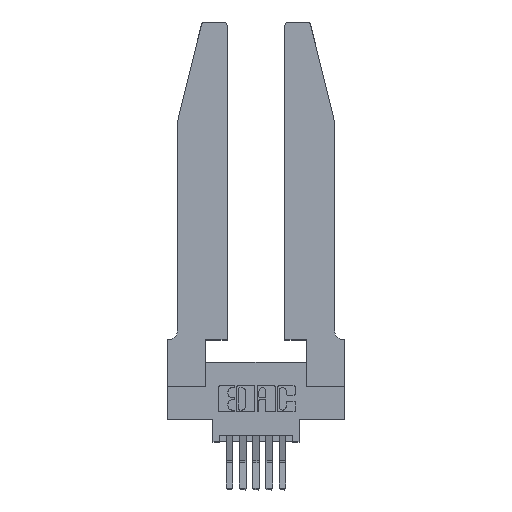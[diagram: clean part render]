
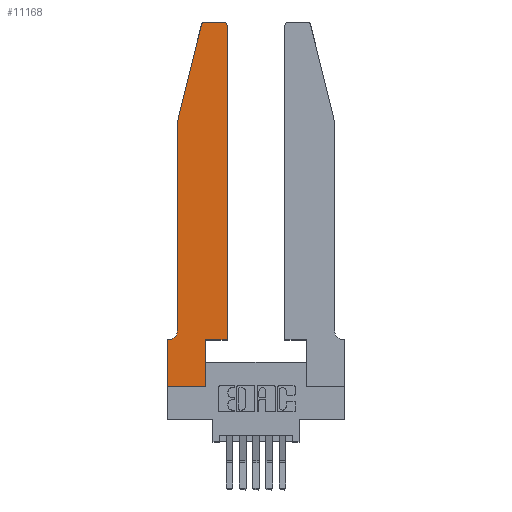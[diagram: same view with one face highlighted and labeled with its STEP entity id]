
A CAD part, top view. The second image highlights one B-rep face of the part: STEP entity #11168.
In plain terms, the highlighted planar face has unit normal (0, 0, 1).
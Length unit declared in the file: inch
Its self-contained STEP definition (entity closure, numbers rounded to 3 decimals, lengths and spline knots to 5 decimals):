
#159 = AXIS2_PLACEMENT_3D ( 'NONE', #1647, #2772, #8067 ) ;
#267 = VECTOR ( 'NONE', #5500, 39.37008 ) ;
#346 = CARTESIAN_POINT ( 'NONE',  ( 0., 0.35, 0.37 ) ) ;
#386 = CARTESIAN_POINT ( 'NONE',  ( 0., 0., 0.37 ) ) ;
#785 = CARTESIAN_POINT ( 'NONE',  ( 0.4205, 2.75, 0.37 ) ) ;
#828 = PLANE ( 'NONE',  #159 ) ;
#939 = ORIENTED_EDGE ( 'NONE', *, *, #6567, .T. ) ;
#1120 = ORIENTED_EDGE ( 'NONE', *, *, #12400, .T. ) ;
#1307 = EDGE_CURVE ( 'NONE', #7925, #9854, #4342, .T. ) ;
#1395 = CARTESIAN_POINT ( 'NONE',  ( 0.4505, 0.35, 0.37 ) ) ;
#1407 = DIRECTION ( 'NONE',  ( 0., 1., 0. ) ) ;
#1647 = CARTESIAN_POINT ( 'NONE',  ( 0., 0.35, 0.37 ) ) ;
#1741 = VERTEX_POINT ( 'NONE', #12977 ) ;
#1859 = AXIS2_PLACEMENT_3D ( 'NONE', #12601, #13687, #10317 ) ;
#1893 = CIRCLE ( 'NONE', #5545, 0.07 ) ;
#1954 = CARTESIAN_POINT ( 'NONE',  ( 0.0755, 0.42, 0.37 ) ) ;
#2406 = ORIENTED_EDGE ( 'NONE', *, *, #13026, .T. ) ;
#2427 = FACE_OUTER_BOUND ( 'NONE', #3702, .T. ) ;
#2658 = VECTOR ( 'NONE', #3907, 39.37008 ) ;
#2772 = DIRECTION ( 'NONE',  ( 0., 0., 1. ) ) ;
#2905 = CARTESIAN_POINT ( 'NONE',  ( 0.0755, 2., 0.37 ) ) ;
#2915 = VECTOR ( 'NONE', #4854, 39.37008 ) ;
#2920 = AXIS2_PLACEMENT_3D ( 'NONE', #3860, #5996, #12474 ) ;
#2990 = ORIENTED_EDGE ( 'NONE', *, *, #1307, .T. ) ;
#3074 = ORIENTED_EDGE ( 'NONE', *, *, #8545, .T. ) ;
#3184 = CARTESIAN_POINT ( 'NONE',  ( 0.4505, 0.35, 0.37 ) ) ;
#3205 = ORIENTED_EDGE ( 'NONE', *, *, #9961, .T. ) ;
#3292 = LINE ( 'NONE', #6955, #13682 ) ;
#3400 = ORIENTED_EDGE ( 'NONE', *, *, #11657, .T. ) ;
#3604 = CARTESIAN_POINT ( 'NONE',  ( 0.2865, 0.35, 0.37 ) ) ;
#3702 = EDGE_LOOP ( 'NONE', ( #10609, #3205, #7312, #8135, #3074, #1120, #2990, #3823, #939, #12648, #2406, #3400 ) ) ;
#3823 = ORIENTED_EDGE ( 'NONE', *, *, #11469, .T. ) ;
#3860 = CARTESIAN_POINT ( 'NONE',  ( 0.284, 2.72, 0.37 ) ) ;
#3907 = DIRECTION ( 'NONE',  ( 0., -1., 0. ) ) ;
#4028 = DIRECTION ( 'NONE',  ( 0., 1., 0. ) ) ;
#4201 = CARTESIAN_POINT ( 'NONE',  ( 0.0055, 0.42, 0.37 ) ) ;
#4342 = LINE ( 'NONE', #8111, #2658 ) ;
#4854 = DIRECTION ( 'NONE',  ( -1., 0., 0. ) ) ;
#5061 = LINE ( 'NONE', #13356, #8101 ) ;
#5265 = CARTESIAN_POINT ( 'NONE',  ( 0.2865, 0.35, 0.37 ) ) ;
#5500 = DIRECTION ( 'NONE',  ( 1., 0., 0. ) ) ;
#5545 = AXIS2_PLACEMENT_3D ( 'NONE', #4201, #5985, #7476 ) ;
#5696 = CARTESIAN_POINT ( 'NONE',  ( 0.0755, 0.35, 0.37 ) ) ;
#5869 = CARTESIAN_POINT ( 'NONE',  ( 0.2605, 2.75, 0.37 ) ) ;
#5920 = VERTEX_POINT ( 'NONE', #1395 ) ;
#5985 = DIRECTION ( 'NONE',  ( 0., 0., -1. ) ) ;
#5996 = DIRECTION ( 'NONE',  ( 0., 0., 1. ) ) ;
#6066 = LINE ( 'NONE', #5696, #12959 ) ;
#6400 = VERTEX_POINT ( 'NONE', #13180 ) ;
#6419 = DIRECTION ( 'NONE',  ( 1., 0., 0. ) ) ;
#6444 = VERTEX_POINT ( 'NONE', #13510 ) ;
#6567 = EDGE_CURVE ( 'NONE', #6400, #8113, #13697, .T. ) ;
#6667 = VERTEX_POINT ( 'NONE', #13475 ) ;
#6842 = EDGE_CURVE ( 'NONE', #11203, #7207, #3292, .T. ) ;
#6850 = CARTESIAN_POINT ( 'NONE',  ( 0.284, 2.75, 0.37 ) ) ;
#6955 = CARTESIAN_POINT ( 'NONE',  ( 0.0755, 2., 0.37 ) ) ;
#7089 = EDGE_CURVE ( 'NONE', #8657, #8095, #8960, .T. ) ;
#7207 = VERTEX_POINT ( 'NONE', #1954 ) ;
#7312 = ORIENTED_EDGE ( 'NONE', *, *, #12575, .T. ) ;
#7476 = DIRECTION ( 'NONE',  ( -1., 0., 0. ) ) ;
#7925 = VERTEX_POINT ( 'NONE', #346 ) ;
#8067 = DIRECTION ( 'NONE',  ( 1., 0., 0. ) ) ;
#8095 = VERTEX_POINT ( 'NONE', #6850 ) ;
#8101 = VECTOR ( 'NONE', #1407, 39.37008 ) ;
#8111 = CARTESIAN_POINT ( 'NONE',  ( 0., 0., 0.37 ) ) ;
#8113 = VERTEX_POINT ( 'NONE', #3604 ) ;
#8119 = LINE ( 'NONE', #8670, #8792 ) ;
#8135 = ORIENTED_EDGE ( 'NONE', *, *, #6842, .T. ) ;
#8545 = EDGE_CURVE ( 'NONE', #7207, #6444, #1893, .T. ) ;
#8657 = VERTEX_POINT ( 'NONE', #785 ) ;
#8670 = CARTESIAN_POINT ( 'NONE',  ( 0., 0., 0.37 ) ) ;
#8792 = VECTOR ( 'NONE', #6419, 39.37008 ) ;
#8960 = LINE ( 'NONE', #5869, #2915 ) ;
#9854 = VERTEX_POINT ( 'NONE', #386 ) ;
#9961 = EDGE_CURVE ( 'NONE', #8095, #6667, #11938, .T. ) ;
#10291 = VECTOR ( 'NONE', #12720, 39.37008 ) ;
#10317 = DIRECTION ( 'NONE',  ( 1., 0., 0. ) ) ;
#10609 = ORIENTED_EDGE ( 'NONE', *, *, #7089, .T. ) ;
#10965 = EDGE_CURVE ( 'NONE', #8113, #5920, #12004, .T. ) ;
#11154 = DIRECTION ( 'NONE',  ( 0., -1., 0. ) ) ;
#11168 = ADVANCED_FACE ( 'NONE', ( #2427 ), #828, .T. ) ;
#11182 = VECTOR ( 'NONE', #4028, 39.37008 ) ;
#11203 = VERTEX_POINT ( 'NONE', #2905 ) ;
#11469 = EDGE_CURVE ( 'NONE', #9854, #6400, #8119, .T. ) ;
#11643 = CIRCLE ( 'NONE', #1859, 0.03 ) ;
#11657 = EDGE_CURVE ( 'NONE', #1741, #8657, #11643, .T. ) ;
#11938 = CIRCLE ( 'NONE', #2920, 0.03 ) ;
#12004 = LINE ( 'NONE', #3184, #267 ) ;
#12065 = DIRECTION ( 'NONE',  ( -1., 0., 0. ) ) ;
#12400 = EDGE_CURVE ( 'NONE', #6444, #7925, #6066, .T. ) ;
#12474 = DIRECTION ( 'NONE',  ( 1., 0., 0. ) ) ;
#12575 = EDGE_CURVE ( 'NONE', #6667, #11203, #13129, .T. ) ;
#12601 = CARTESIAN_POINT ( 'NONE',  ( 0.4205, 2.72, 0.37 ) ) ;
#12648 = ORIENTED_EDGE ( 'NONE', *, *, #10965, .T. ) ;
#12720 = DIRECTION ( 'NONE',  ( -0.239, -0.971, 0. ) ) ;
#12959 = VECTOR ( 'NONE', #12065, 39.37008 ) ;
#12977 = CARTESIAN_POINT ( 'NONE',  ( 0.4505, 2.72, 0.37 ) ) ;
#13026 = EDGE_CURVE ( 'NONE', #5920, #1741, #5061, .T. ) ;
#13129 = LINE ( 'NONE', #13708, #10291 ) ;
#13180 = CARTESIAN_POINT ( 'NONE',  ( 0.2865, 0., 0.37 ) ) ;
#13356 = CARTESIAN_POINT ( 'NONE',  ( 0.4505, 0.35, 0.37 ) ) ;
#13475 = CARTESIAN_POINT ( 'NONE',  ( 0.25487, 2.72718, 0.37 ) ) ;
#13510 = CARTESIAN_POINT ( 'NONE',  ( 0.0055, 0.35, 0.37 ) ) ;
#13682 = VECTOR ( 'NONE', #11154, 39.37008 ) ;
#13687 = DIRECTION ( 'NONE',  ( 0., 0., 1. ) ) ;
#13697 = LINE ( 'NONE', #5265, #11182 ) ;
#13708 = CARTESIAN_POINT ( 'NONE',  ( 0.0755, 2., 0.37 ) ) ;
